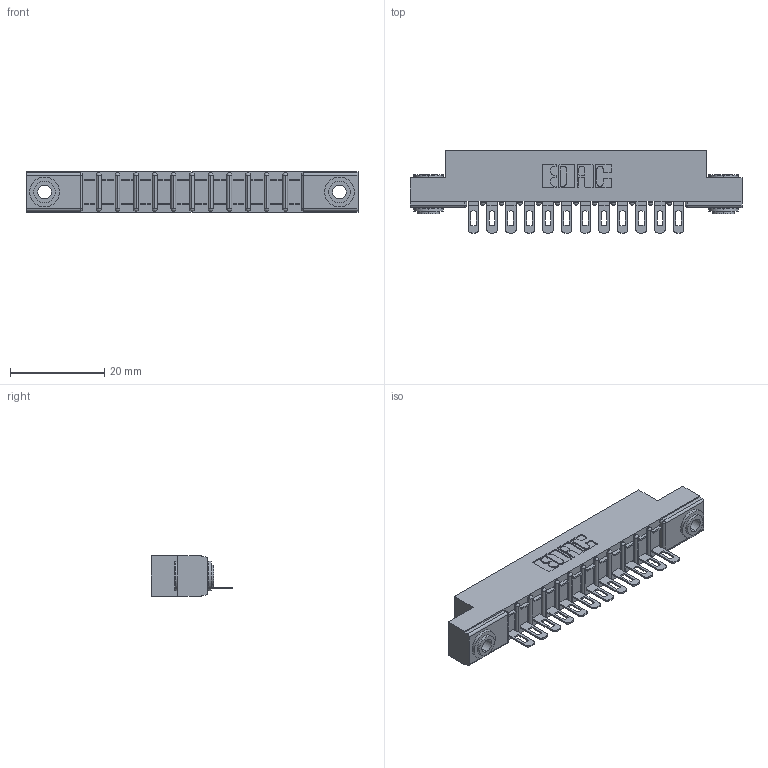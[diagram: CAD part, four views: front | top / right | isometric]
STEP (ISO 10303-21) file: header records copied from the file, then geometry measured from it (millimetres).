
FILE_DESCRIPTION (( 'STEP AP203' ), '1' );
FILE_NAME ('307-012-501-103.STEP', '2019-09-04T19:42:47', ( '' ), ( '' ), 'SwSTEP 2.0', 'SolidWorks 2016', '' );
FILE_SCHEMA (( 'CONFIG_CONTROL_DESIGN' ));
Length unit declared in the file: inch
Products named in the file (4): 307-012-501-103; 345-250-002_345-250-002-102; 307-290-002_501; 307 Part_.156 Dia Mounting Holes
Assembly tree (15 placements, depth 2):
  307-012-501-103
    307 Part_.156 Dia Mounting Holes
    307-290-002_501  x12
    345-250-002_345-250-002-102  x2
Bounding box: 70.56 x 17.42 x 8.71 mm (x, y, z)
Volume: 4664.8 mm3; surface area: 8253.2 mm2
Topology: 15 solids, 15 shells, 1095 faces, 3291 edges, 2154 vertices
Faces by surface type: plane 622, cylinder 439, sphere 26, cone 8
Entity records: 15845 total; most frequent: CARTESIAN_POINT 2645, ORIENTED_EDGE 2626, DIRECTION 2603, EDGE_CURVE 1313, VECTOR 979, LINE 979, VERTEX_POINT 854, AXIS2_PLACEMENT_3D 812
